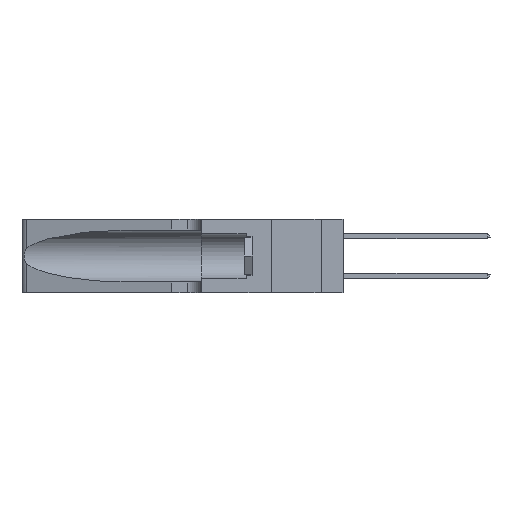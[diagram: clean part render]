
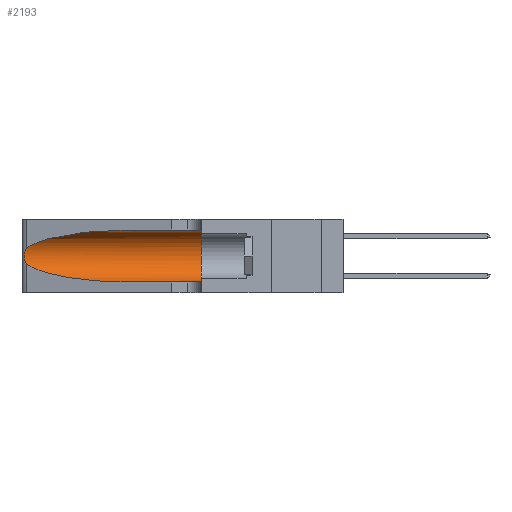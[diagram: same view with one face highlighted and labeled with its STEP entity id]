
A CAD part, left-side view. The second image highlights one B-rep face of the part: STEP entity #2193.
In plain terms, the highlighted cylindrical face has radius 3.308 mm (diameter 6.617 mm), a partial arc.
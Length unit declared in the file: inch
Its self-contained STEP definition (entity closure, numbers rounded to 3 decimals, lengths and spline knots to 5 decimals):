
#79 = CARTESIAN_POINT ( 'NONE',  ( 0.1305, 1.61858, 0.31525 ) ) ;
#894 = CARTESIAN_POINT ( 'NONE',  ( 0.25555, 1.22993, 0.14849 ) ) ;
#1638 = VERTEX_POINT ( 'NONE', #20291 ) ;
#2193 = ADVANCED_FACE ( 'NONE', ( #7433 ), #6256, .F. ) ;
#2546 = VECTOR ( 'NONE', #3074, 39.37008 ) ;
#2974 = EDGE_CURVE ( 'NONE', #6182, #26332, #9443, .T. ) ;
#3074 = DIRECTION ( 'NONE',  ( 0., -1., 0. ) ) ;
#3557 = ORIENTED_EDGE ( 'NONE', *, *, #21893, .F. ) ;
#3914 = ORIENTED_EDGE ( 'NONE', *, *, #24782, .T. ) ;
#3988 = CARTESIAN_POINT ( 'NONE',  ( 0.1305, 0.72297, 0.31525 ) ) ;
#4317 = CARTESIAN_POINT ( 'NONE',  ( 0.1305, 0.35, 0.185 ) ) ;
#5157 = CARTESIAN_POINT ( 'NONE',  ( 0.1305, 1.61858, 0.185 ) ) ;
#5988 = CARTESIAN_POINT ( 'NONE',  ( 0.25787, 1.23484, 0.2124 ) ) ;
#6182 = VERTEX_POINT ( 'NONE', #26871 ) ;
#6256 = CYLINDRICAL_SURFACE ( 'NONE', #16801, 0.13025 ) ;
#6948 = DIRECTION ( 'NONE',  ( 0., 0., 1. ) ) ;
#7233 = CARTESIAN_POINT ( 'NONE',  ( 0.1305, 0.72297, 0.31525 ) ) ;
#7433 = FACE_OUTER_BOUND ( 'NONE', #8687, .T. ) ;
#8612 = CARTESIAN_POINT ( 'NONE',  ( 0.26018, 1.23835, 0.19895 ) ) ;
#8687 = EDGE_LOOP ( 'NONE', ( #3914, #26698, #12799, #25614, #13062, #3557 ) ) ;
#9443 = LINE ( 'NONE', #30534, #2546 ) ;
#9480 = VERTEX_POINT ( 'NONE', #25987 ) ;
#10834 =( BOUNDED_CURVE ( )  B_SPLINE_CURVE ( 3, ( #3988, #19124, #11770, #29003 ),
 .UNSPECIFIED., .F., .T. ) 
 B_SPLINE_CURVE_WITH_KNOTS ( ( 4, 4 ),
 ( 1.5708, 2.84003 ),
 .UNSPECIFIED. ) 
 CURVE ( )  GEOMETRIC_REPRESENTATION_ITEM ( )  RATIONAL_B_SPLINE_CURVE ( ( 1., 0.87, 0.87, 1. ) ) 
 REPRESENTATION_ITEM ( '' )  );
#11166 = CARTESIAN_POINT ( 'NONE',  ( 0.26075, 1.23896, 0.178 ) ) ;
#11770 = CARTESIAN_POINT ( 'NONE',  ( 0.2373, 1.15595, 0.28018 ) ) ;
#12144 = CARTESIAN_POINT ( 'NONE',  ( 0.18966, 0.96281, 0.05475 ) ) ;
#12799 = ORIENTED_EDGE ( 'NONE', *, *, #18582, .T. ) ;
#13062 = ORIENTED_EDGE ( 'NONE', *, *, #15331, .F. ) ;
#13268 = B_SPLINE_CURVE_WITH_KNOTS ( 'NONE', 3,
 ( #18549, #30837, #21032, #5988, #23509, #8612, #25949, #11166, #28436, #13704, #30943, #16190, #894, #18657 ),
 .UNSPECIFIED., .F., .F.,
 ( 4, 2, 2, 2, 2, 2, 4 ),
 ( 0., 0.00027, 0.00053, 0.00107, 0.0016, 0.00187, 0.00214 ),
 .UNSPECIFIED. ) ;
#13704 = CARTESIAN_POINT ( 'NONE',  ( 0.25856, 1.23593, 0.16098 ) ) ;
#13876 = EDGE_CURVE ( 'NONE', #1638, #21651, #13268, .T. ) ;
#14221 = VERTEX_POINT ( 'NONE', #7233 ) ;
#15331 = EDGE_CURVE ( 'NONE', #9480, #26332, #29856, .T. ) ;
#16190 = CARTESIAN_POINT ( 'NONE',  ( 0.25639, 1.23186, 0.15144 ) ) ;
#16801 = AXIS2_PLACEMENT_3D ( 'NONE', #5157, #25174, #20259 ) ;
#17898 = DIRECTION ( 'NONE',  ( 0., -1., 0. ) ) ;
#18549 = CARTESIAN_POINT ( 'NONE',  ( 0.25487, 1.22718, 0.22369 ) ) ;
#18582 = EDGE_CURVE ( 'NONE', #21651, #6182, #22364, .T. ) ;
#18657 = CARTESIAN_POINT ( 'NONE',  ( 0.25487, 1.22718, 0.14631 ) ) ;
#19124 = CARTESIAN_POINT ( 'NONE',  ( 0.18966, 0.96281, 0.31525 ) ) ;
#20259 = DIRECTION ( 'NONE',  ( 0., 0., -1. ) ) ;
#20291 = CARTESIAN_POINT ( 'NONE',  ( 0.25487, 1.22718, 0.22369 ) ) ;
#21032 = CARTESIAN_POINT ( 'NONE',  ( 0.25639, 1.23184, 0.21858 ) ) ;
#21651 = VERTEX_POINT ( 'NONE', #24891 ) ;
#21877 = VECTOR ( 'NONE', #17898, 39.37008 ) ;
#21893 = EDGE_CURVE ( 'NONE', #14221, #9480, #28389, .T. ) ;
#21931 = DIRECTION ( 'NONE',  ( 0., 1., 0. ) ) ;
#22364 =( BOUNDED_CURVE ( )  B_SPLINE_CURVE ( 3, ( #24410, #26886, #12144, #29368 ),
 .UNSPECIFIED., .F., .F. ) 
 B_SPLINE_CURVE_WITH_KNOTS ( ( 4, 4 ),
 ( 3.44316, 4.71239 ),
 .UNSPECIFIED. ) 
 CURVE ( )  GEOMETRIC_REPRESENTATION_ITEM ( )  RATIONAL_B_SPLINE_CURVE ( ( 1., 0.87, 0.87, 1. ) ) 
 REPRESENTATION_ITEM ( '' )  );
#23509 = CARTESIAN_POINT ( 'NONE',  ( 0.25854, 1.2359, 0.20912 ) ) ;
#23756 = CARTESIAN_POINT ( 'NONE',  ( 0.1305, 0.35, 0.05475 ) ) ;
#24410 = CARTESIAN_POINT ( 'NONE',  ( 0.25487, 1.22718, 0.14631 ) ) ;
#24782 = EDGE_CURVE ( 'NONE', #14221, #1638, #10834, .T. ) ;
#24891 = CARTESIAN_POINT ( 'NONE',  ( 0.25487, 1.22718, 0.14631 ) ) ;
#25174 = DIRECTION ( 'NONE',  ( 0., -1., 0. ) ) ;
#25614 = ORIENTED_EDGE ( 'NONE', *, *, #2974, .T. ) ;
#25949 = CARTESIAN_POINT ( 'NONE',  ( 0.26075, 1.23896, 0.19203 ) ) ;
#25987 = CARTESIAN_POINT ( 'NONE',  ( 0.1305, 0.35, 0.31525 ) ) ;
#26332 = VERTEX_POINT ( 'NONE', #23756 ) ;
#26698 = ORIENTED_EDGE ( 'NONE', *, *, #13876, .T. ) ;
#26871 = CARTESIAN_POINT ( 'NONE',  ( 0.1305, 0.72297, 0.05475 ) ) ;
#26886 = CARTESIAN_POINT ( 'NONE',  ( 0.2373, 1.15595, 0.08982 ) ) ;
#28389 = LINE ( 'NONE', #79, #21877 ) ;
#28436 = CARTESIAN_POINT ( 'NONE',  ( 0.26017, 1.23833, 0.17102 ) ) ;
#29003 = CARTESIAN_POINT ( 'NONE',  ( 0.25487, 1.22718, 0.22369 ) ) ;
#29368 = CARTESIAN_POINT ( 'NONE',  ( 0.1305, 0.72297, 0.05475 ) ) ;
#29856 = CIRCLE ( 'NONE', #30854, 0.13025 ) ;
#30534 = CARTESIAN_POINT ( 'NONE',  ( 0.1305, 1.61858, 0.05475 ) ) ;
#30837 = CARTESIAN_POINT ( 'NONE',  ( 0.25555, 1.22994, 0.2215 ) ) ;
#30854 = AXIS2_PLACEMENT_3D ( 'NONE', #4317, #21931, #6948 ) ;
#30943 = CARTESIAN_POINT ( 'NONE',  ( 0.25789, 1.23486, 0.15765 ) ) ;
